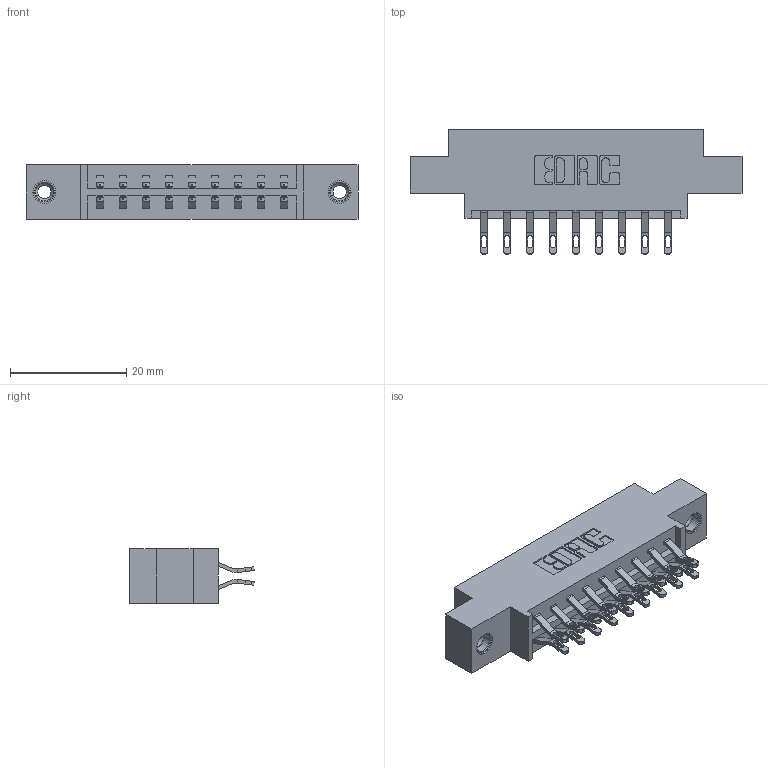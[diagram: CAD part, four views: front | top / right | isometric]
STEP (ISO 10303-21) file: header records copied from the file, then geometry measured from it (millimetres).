
FILE_DESCRIPTION (( 'STEP AP203' ), '1' );
FILE_NAME ('333-018-555-808.STEP', '2019-08-09T14:00:47', ( '' ), ( '' ), 'SwSTEP 2.0', 'SolidWorks 2016', '' );
FILE_SCHEMA (( 'CONFIG_CONTROL_DESIGN' ));
Length unit declared in the file: inch
Products named in the file (4): 345-250-001_345-250-003-102; 345-292-001_555 Tail; 333-018-555-808; 333 Part_Offset - .156 Dia - TI
Assembly tree (21 placements, depth 2):
  333-018-555-808
    333 Part_Offset - .156 Dia - TI
    345-292-001_555 Tail  x18
    345-250-001_345-250-003-102  x2
Bounding box: 57.2 x 21.47 x 9.4 mm (x, y, z)
Volume: 5349.2 mm3; surface area: 6407.3 mm2
Topology: 21 solids, 21 shells, 1222 faces, 3753 edges, 2494 vertices
Faces by surface type: plane 718, cylinder 488, cone 12, torus 4
Entity records: 11702 total; most frequent: CARTESIAN_POINT 1999, ORIENTED_EDGE 1898, DIRECTION 1767, EDGE_CURVE 949, VECTOR 781, LINE 781, VERTEX_POINT 628, AXIS2_PLACEMENT_3D 493
